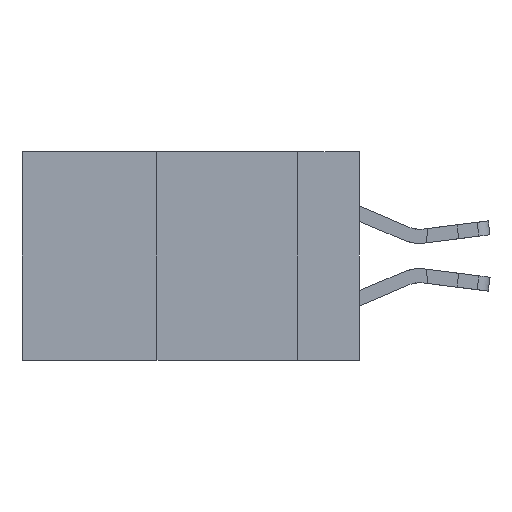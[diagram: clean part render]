
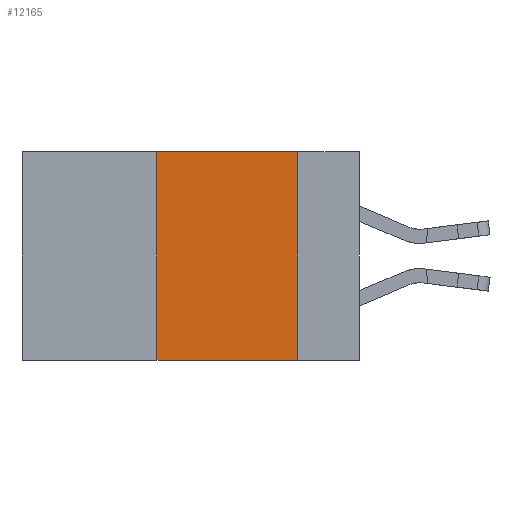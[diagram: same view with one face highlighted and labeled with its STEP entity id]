
A CAD part, left-side view. The second image highlights one B-rep face of the part: STEP entity #12165.
In plain terms, the highlighted planar face has unit normal (-1, 0, 0).
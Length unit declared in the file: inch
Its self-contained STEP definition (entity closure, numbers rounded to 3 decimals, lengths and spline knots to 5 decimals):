
#78 = DIRECTION ( 'NONE',  ( 1., 0., 0. ) ) ;
#203 = VECTOR ( 'NONE', #15085, 39.37008 ) ;
#816 = LINE ( 'NONE', #9310, #8343 ) ;
#938 = ORIENTED_EDGE ( 'NONE', *, *, #8858, .T. ) ;
#1334 = DIRECTION ( 'NONE',  ( 0., -1., 0. ) ) ;
#1550 = CARTESIAN_POINT ( 'NONE',  ( 0., 0.6, 0. ) ) ;
#1559 = VERTEX_POINT ( 'NONE', #4668 ) ;
#3068 = ORIENTED_EDGE ( 'NONE', *, *, #7751, .F. ) ;
#4175 = VERTEX_POINT ( 'NONE', #4579 ) ;
#4203 = VERTEX_POINT ( 'NONE', #15308 ) ;
#4579 = CARTESIAN_POINT ( 'NONE',  ( 0., 0.36, -0.37 ) ) ;
#4668 = CARTESIAN_POINT ( 'NONE',  ( 0., 0.11, 0. ) ) ;
#6608 = VERTEX_POINT ( 'NONE', #9879 ) ;
#6847 = VECTOR ( 'NONE', #1334, 39.37008 ) ;
#7751 = EDGE_CURVE ( 'NONE', #4175, #6608, #816, .T. ) ;
#8301 = VECTOR ( 'NONE', #11588, 39.37008 ) ;
#8343 = VECTOR ( 'NONE', #15279, 39.37008 ) ;
#8413 = EDGE_LOOP ( 'NONE', ( #10531, #9143, #3068, #938 ) ) ;
#8858 = EDGE_CURVE ( 'NONE', #4175, #4203, #18429, .T. ) ;
#9143 = ORIENTED_EDGE ( 'NONE', *, *, #14907, .F. ) ;
#9310 = CARTESIAN_POINT ( 'NONE',  ( 0., 0.36, 0. ) ) ;
#9879 = CARTESIAN_POINT ( 'NONE',  ( 0., 0.36, 0. ) ) ;
#10066 = CARTESIAN_POINT ( 'NONE',  ( 0., 0.11, 0. ) ) ;
#10531 = ORIENTED_EDGE ( 'NONE', *, *, #17976, .F. ) ;
#10606 = DIRECTION ( 'NONE',  ( 0., 0., -1. ) ) ;
#11588 = DIRECTION ( 'NONE',  ( 0., 0., -1. ) ) ;
#12165 = ADVANCED_FACE ( 'NONE', ( #13955 ), #16402, .F. ) ;
#12540 = AXIS2_PLACEMENT_3D ( 'NONE', #1550, #78, #10606 ) ;
#12737 = LINE ( 'NONE', #10066, #8301 ) ;
#13312 = CARTESIAN_POINT ( 'NONE',  ( 0., 0.6, -0.37 ) ) ;
#13955 = FACE_OUTER_BOUND ( 'NONE', #8413, .T. ) ;
#14907 = EDGE_CURVE ( 'NONE', #6608, #1559, #15635, .T. ) ;
#15085 = DIRECTION ( 'NONE',  ( 0., -1., 0. ) ) ;
#15279 = DIRECTION ( 'NONE',  ( 0., 0., 1. ) ) ;
#15308 = CARTESIAN_POINT ( 'NONE',  ( 0., 0.11, -0.37 ) ) ;
#15635 = LINE ( 'NONE', #17849, #203 ) ;
#16402 = PLANE ( 'NONE',  #12540 ) ;
#17849 = CARTESIAN_POINT ( 'NONE',  ( 0., 0.6, 0. ) ) ;
#17976 = EDGE_CURVE ( 'NONE', #1559, #4203, #12737, .T. ) ;
#18429 = LINE ( 'NONE', #13312, #6847 ) ;
